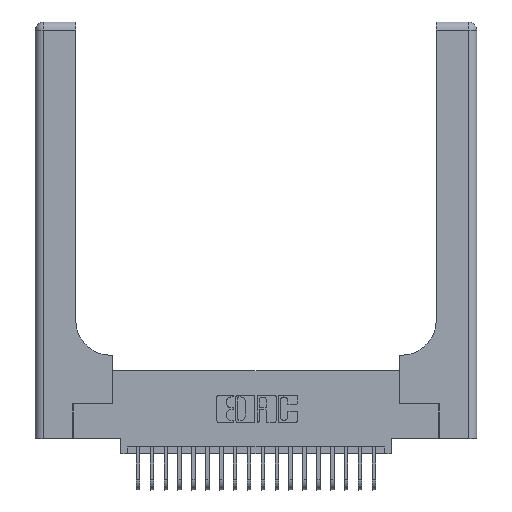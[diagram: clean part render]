
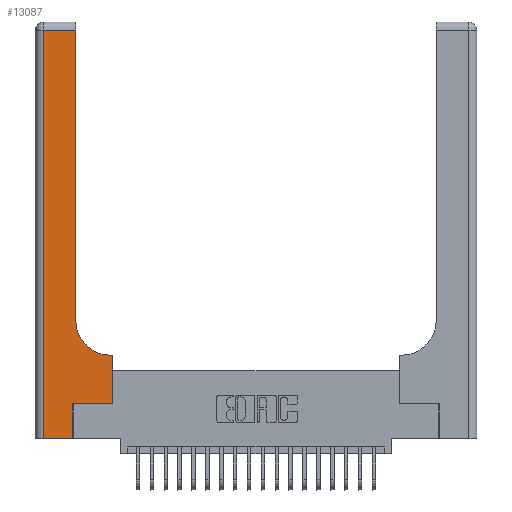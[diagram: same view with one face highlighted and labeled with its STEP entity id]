
A CAD part, top view. The second image highlights one B-rep face of the part: STEP entity #13087.
In plain terms, the highlighted planar face has unit normal (0, 0, 1).
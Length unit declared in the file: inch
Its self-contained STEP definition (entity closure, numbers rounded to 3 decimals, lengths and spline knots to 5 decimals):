
#696 = CIRCLE ( 'NONE', #9935, 0.25 ) ;
#1468 = LINE ( 'NONE', #2598, #13671 ) ;
#1550 = CARTESIAN_POINT ( 'NONE',  ( 0.2915, 0.85, 0.37 ) ) ;
#2121 = VERTEX_POINT ( 'NONE', #1550 ) ;
#2127 = DIRECTION ( 'NONE',  ( 0., 0., -1. ) ) ;
#2329 = DIRECTION ( 'NONE',  ( 1., 0., 0. ) ) ;
#2346 = CARTESIAN_POINT ( 'NONE',  ( 0.06, 0., 0.37 ) ) ;
#2598 = CARTESIAN_POINT ( 'NONE',  ( 0.2915, 0.6, 0.37 ) ) ;
#2808 = EDGE_CURVE ( 'NONE', #6211, #10631, #12377, .T. ) ;
#2946 = EDGE_CURVE ( 'NONE', #10424, #5001, #1468, .T. ) ;
#3159 = EDGE_CURVE ( 'NONE', #11049, #4990, #11041, .T. ) ;
#3485 = CARTESIAN_POINT ( 'NONE',  ( 0.269, 0.25, 0.37 ) ) ;
#3659 = EDGE_CURVE ( 'NONE', #4990, #10424, #16557, .T. ) ;
#3979 = CARTESIAN_POINT ( 'NONE',  ( 0.2915, 3., 0.37 ) ) ;
#4102 = CARTESIAN_POINT ( 'NONE',  ( 0., 0., 0.37 ) ) ;
#4340 = CARTESIAN_POINT ( 'NONE',  ( 0.5585, 0.25, 0.37 ) ) ;
#4375 = LINE ( 'NONE', #4102, #13032 ) ;
#4612 = PLANE ( 'NONE',  #6913 ) ;
#4871 = VECTOR ( 'NONE', #21292, 39.37008 ) ;
#4990 = VERTEX_POINT ( 'NONE', #19841 ) ;
#5001 = VERTEX_POINT ( 'NONE', #9701 ) ;
#5303 = ORIENTED_EDGE ( 'NONE', *, *, #2808, .T. ) ;
#5321 = ORIENTED_EDGE ( 'NONE', *, *, #7338, .T. ) ;
#5404 = CARTESIAN_POINT ( 'NONE',  ( 0.06, 3., 0.37 ) ) ;
#5908 = ORIENTED_EDGE ( 'NONE', *, *, #21519, .T. ) ;
#6110 = ORIENTED_EDGE ( 'NONE', *, *, #3659, .T. ) ;
#6186 = VERTEX_POINT ( 'NONE', #10993 ) ;
#6211 = VERTEX_POINT ( 'NONE', #11133 ) ;
#6913 = AXIS2_PLACEMENT_3D ( 'NONE', #14895, #19963, #9829 ) ;
#6981 = VECTOR ( 'NONE', #16053, 39.37008 ) ;
#7204 = FACE_OUTER_BOUND ( 'NONE', #12431, .T. ) ;
#7338 = EDGE_CURVE ( 'NONE', #10631, #8108, #7423, .T. ) ;
#7423 = LINE ( 'NONE', #5404, #19903 ) ;
#8089 = ORIENTED_EDGE ( 'NONE', *, *, #8649, .T. ) ;
#8108 = VERTEX_POINT ( 'NONE', #2346 ) ;
#8158 = ORIENTED_EDGE ( 'NONE', *, *, #10695, .T. ) ;
#8559 = ORIENTED_EDGE ( 'NONE', *, *, #3159, .T. ) ;
#8649 = EDGE_CURVE ( 'NONE', #8108, #6186, #4375, .T. ) ;
#9213 = ORIENTED_EDGE ( 'NONE', *, *, #2946, .T. ) ;
#9562 = DIRECTION ( 'NONE',  ( 0., 1., 0. ) ) ;
#9701 = CARTESIAN_POINT ( 'NONE',  ( 0.5415, 0.6, 0.37 ) ) ;
#9829 = DIRECTION ( 'NONE',  ( -1., 0., 0. ) ) ;
#9935 = AXIS2_PLACEMENT_3D ( 'NONE', #12538, #2127, #14220 ) ;
#9971 = CARTESIAN_POINT ( 'NONE',  ( 0.269, 0.25, 0.37 ) ) ;
#10424 = VERTEX_POINT ( 'NONE', #13906 ) ;
#10491 = VECTOR ( 'NONE', #15096, 39.37008 ) ;
#10631 = VERTEX_POINT ( 'NONE', #17776 ) ;
#10695 = EDGE_CURVE ( 'NONE', #6186, #11049, #13487, .T. ) ;
#10993 = CARTESIAN_POINT ( 'NONE',  ( 0.269, 0., 0.37 ) ) ;
#11041 = LINE ( 'NONE', #9971, #10491 ) ;
#11049 = VERTEX_POINT ( 'NONE', #3485 ) ;
#11133 = CARTESIAN_POINT ( 'NONE',  ( 0.2915, 2.94, 0.37 ) ) ;
#11589 = LINE ( 'NONE', #3979, #6981 ) ;
#12109 = VECTOR ( 'NONE', #9562, 39.37008 ) ;
#12377 = LINE ( 'NONE', #17443, #16302 ) ;
#12431 = EDGE_LOOP ( 'NONE', ( #5908, #5303, #5321, #8089, #8158, #8559, #6110, #9213, #22154 ) ) ;
#12538 = CARTESIAN_POINT ( 'NONE',  ( 0.5415, 0.85, 0.37 ) ) ;
#12916 = DIRECTION ( 'NONE',  ( -1., 0., 0. ) ) ;
#12952 = CARTESIAN_POINT ( 'NONE',  ( 0.269, 0., 0.37 ) ) ;
#13032 = VECTOR ( 'NONE', #2329, 39.37008 ) ;
#13087 = ADVANCED_FACE ( 'NONE', ( #7204 ), #4612, .F. ) ;
#13487 = LINE ( 'NONE', #12952, #4871 ) ;
#13514 = EDGE_CURVE ( 'NONE', #5001, #2121, #696, .T. ) ;
#13671 = VECTOR ( 'NONE', #12916, 39.37008 ) ;
#13906 = CARTESIAN_POINT ( 'NONE',  ( 0.5585, 0.6, 0.37 ) ) ;
#14220 = DIRECTION ( 'NONE',  ( 1., 0., 0. ) ) ;
#14895 = CARTESIAN_POINT ( 'NONE',  ( 0., 3., 0.37 ) ) ;
#15096 = DIRECTION ( 'NONE',  ( 1., 0., 0. ) ) ;
#15778 = DIRECTION ( 'NONE',  ( -1., 0., 0. ) ) ;
#16053 = DIRECTION ( 'NONE',  ( 0., 1., 0. ) ) ;
#16302 = VECTOR ( 'NONE', #15778, 39.37008 ) ;
#16557 = LINE ( 'NONE', #4340, #12109 ) ;
#17443 = CARTESIAN_POINT ( 'NONE',  ( 0., 2.94, 0.37 ) ) ;
#17776 = CARTESIAN_POINT ( 'NONE',  ( 0.06, 2.94, 0.37 ) ) ;
#19841 = CARTESIAN_POINT ( 'NONE',  ( 0.5585, 0.25, 0.37 ) ) ;
#19903 = VECTOR ( 'NONE', #20623, 39.37008 ) ;
#19963 = DIRECTION ( 'NONE',  ( 0., 0., -1. ) ) ;
#20623 = DIRECTION ( 'NONE',  ( 0., -1., 0. ) ) ;
#21292 = DIRECTION ( 'NONE',  ( 0., 1., 0. ) ) ;
#21519 = EDGE_CURVE ( 'NONE', #2121, #6211, #11589, .T. ) ;
#22154 = ORIENTED_EDGE ( 'NONE', *, *, #13514, .T. ) ;
